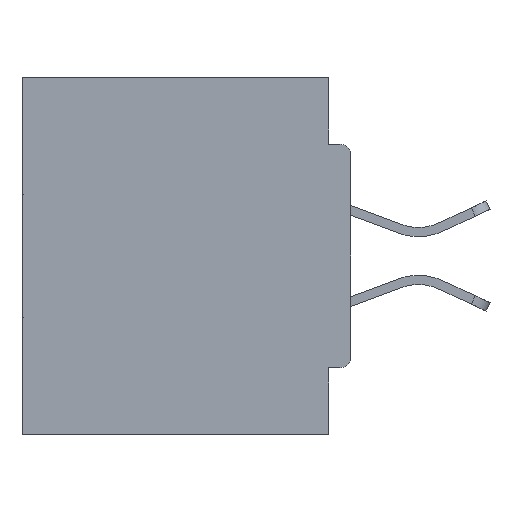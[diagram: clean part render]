
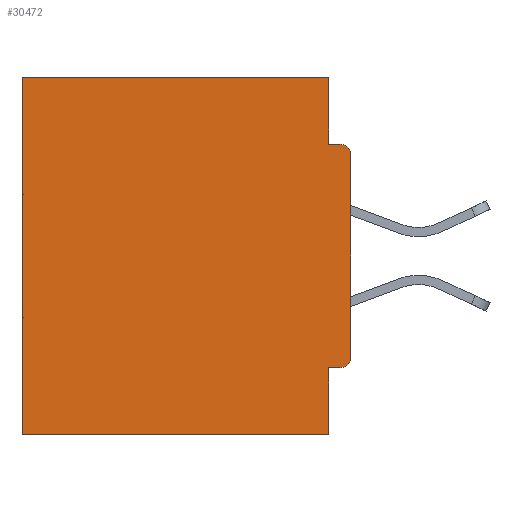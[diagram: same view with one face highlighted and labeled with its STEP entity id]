
A CAD part, left-side view. The second image highlights one B-rep face of the part: STEP entity #30472.
In plain terms, the highlighted planar face has unit normal (-1, 0, 0).
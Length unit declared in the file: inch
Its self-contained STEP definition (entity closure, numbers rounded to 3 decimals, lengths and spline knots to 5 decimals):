
#907 = CARTESIAN_POINT ( 'NONE',  ( 0.298, 0., -0.3915 ) ) ;
#1458 = DIRECTION ( 'NONE',  ( 0., 1., 0. ) ) ;
#2212 = CARTESIAN_POINT ( 'NONE',  ( 0.298, 0.46, 0. ) ) ;
#2393 = CARTESIAN_POINT ( 'NONE',  ( 0.298, 0., -0.1085 ) ) ;
#3038 = CARTESIAN_POINT ( 'NONE',  ( 0.298, 0.015, -0.3915 ) ) ;
#3101 = EDGE_CURVE ( 'NONE', #22892, #24254, #41037, .T. ) ;
#3118 = LINE ( 'NONE', #23529, #28867 ) ;
#4680 = DIRECTION ( 'NONE',  ( 0., 1., 0. ) ) ;
#4734 = EDGE_CURVE ( 'NONE', #29090, #37944, #10026, .T. ) ;
#5075 = DIRECTION ( 'NONE',  ( 0., 0., -1. ) ) ;
#5515 = CIRCLE ( 'NONE', #8658, 0.015 ) ;
#5885 = ORIENTED_EDGE ( 'NONE', *, *, #31345, .F. ) ;
#6039 = CIRCLE ( 'NONE', #16067, 0.015 ) ;
#6059 = CARTESIAN_POINT ( 'NONE',  ( 0.298, 0., 0. ) ) ;
#6969 = CARTESIAN_POINT ( 'NONE',  ( 0.298, 0., 0. ) ) ;
#8136 = CARTESIAN_POINT ( 'NONE',  ( 0.298, 0.015, -0.4065 ) ) ;
#8409 = CARTESIAN_POINT ( 'NONE',  ( 0.298, 0.031, -0.5 ) ) ;
#8658 = AXIS2_PLACEMENT_3D ( 'NONE', #3038, #28784, #19251 ) ;
#8684 = CARTESIAN_POINT ( 'NONE',  ( 0.298, 0.031, -0.4065 ) ) ;
#9141 = VECTOR ( 'NONE', #19854, 39.37008 ) ;
#9294 = CARTESIAN_POINT ( 'NONE',  ( 0.298, 0.015, -0.1085 ) ) ;
#9324 = DIRECTION ( 'NONE',  ( 0., 0., -1. ) ) ;
#9918 = CARTESIAN_POINT ( 'NONE',  ( 0.298, 0.031, -0.5 ) ) ;
#10026 = LINE ( 'NONE', #22534, #19317 ) ;
#10272 = ORIENTED_EDGE ( 'NONE', *, *, #3101, .F. ) ;
#10493 = VERTEX_POINT ( 'NONE', #907 ) ;
#12898 = CARTESIAN_POINT ( 'NONE',  ( 0.298, 0., 0. ) ) ;
#12984 = EDGE_CURVE ( 'NONE', #40757, #29732, #6039, .T. ) ;
#13037 = DIRECTION ( 'NONE',  ( 0., 1., 0. ) ) ;
#13090 = ORIENTED_EDGE ( 'NONE', *, *, #30831, .F. ) ;
#13136 = EDGE_CURVE ( 'NONE', #22892, #10493, #5515, .T. ) ;
#13791 = VECTOR ( 'NONE', #9324, 39.37008 ) ;
#14274 = CARTESIAN_POINT ( 'NONE',  ( 0.298, 0., -0.4065 ) ) ;
#15206 = DIRECTION ( 'NONE',  ( -1., 0., 0. ) ) ;
#15630 = CARTESIAN_POINT ( 'NONE',  ( 0.298, 0.015, -0.0935 ) ) ;
#16067 = AXIS2_PLACEMENT_3D ( 'NONE', #9294, #15206, #41943 ) ;
#16586 = DIRECTION ( 'NONE',  ( 0., 0., -1. ) ) ;
#17011 = PLANE ( 'NONE',  #21272 ) ;
#17064 = ORIENTED_EDGE ( 'NONE', *, *, #37421, .T. ) ;
#17360 = LINE ( 'NONE', #9918, #9141 ) ;
#17787 = ORIENTED_EDGE ( 'NONE', *, *, #29115, .F. ) ;
#17821 = ORIENTED_EDGE ( 'NONE', *, *, #20312, .F. ) ;
#19251 = DIRECTION ( 'NONE',  ( 0., 0., -1. ) ) ;
#19317 = VECTOR ( 'NONE', #31996, 39.37008 ) ;
#19500 = CARTESIAN_POINT ( 'NONE',  ( 0.298, 0.46, -0.5 ) ) ;
#19854 = DIRECTION ( 'NONE',  ( 0., 0., -1. ) ) ;
#20312 = EDGE_CURVE ( 'NONE', #24254, #35761, #17360, .T. ) ;
#21272 = AXIS2_PLACEMENT_3D ( 'NONE', #6969, #29721, #16586 ) ;
#22534 = CARTESIAN_POINT ( 'NONE',  ( 0.298, 0.46, 0. ) ) ;
#22892 = VERTEX_POINT ( 'NONE', #8136 ) ;
#22915 = VERTEX_POINT ( 'NONE', #27572 ) ;
#23529 = CARTESIAN_POINT ( 'NONE',  ( 0.298, 0., -0.0935 ) ) ;
#24254 = VERTEX_POINT ( 'NONE', #8684 ) ;
#24316 = CARTESIAN_POINT ( 'NONE',  ( 0.298, 0., -0.5 ) ) ;
#24353 = ORIENTED_EDGE ( 'NONE', *, *, #36372, .F. ) ;
#24803 = CARTESIAN_POINT ( 'NONE',  ( 0.298, 0.031, -0.5 ) ) ;
#26842 = DIRECTION ( 'NONE',  ( 0., -1., 0. ) ) ;
#27101 = ORIENTED_EDGE ( 'NONE', *, *, #4734, .T. ) ;
#27228 = LINE ( 'NONE', #12898, #32347 ) ;
#27572 = CARTESIAN_POINT ( 'NONE',  ( 0.298, 0.031, -0.0935 ) ) ;
#28109 = FACE_OUTER_BOUND ( 'NONE', #30601, .T. ) ;
#28784 = DIRECTION ( 'NONE',  ( -1., 0., 0. ) ) ;
#28867 = VECTOR ( 'NONE', #26842, 39.37008 ) ;
#29090 = VERTEX_POINT ( 'NONE', #2212 ) ;
#29115 = EDGE_CURVE ( 'NONE', #40757, #10493, #29824, .T. ) ;
#29721 = DIRECTION ( 'NONE',  ( 1., 0., 0. ) ) ;
#29732 = VERTEX_POINT ( 'NONE', #15630 ) ;
#29824 = LINE ( 'NONE', #6059, #13791 ) ;
#30472 = ADVANCED_FACE ( 'NONE', ( #28109 ), #17011, .F. ) ;
#30561 = LINE ( 'NONE', #24316, #39222 ) ;
#30601 = EDGE_LOOP ( 'NONE', ( #40953, #24353, #13090, #17064, #27101, #5885, #17821, #10272, #41126, #17787 ) ) ;
#30831 = EDGE_CURVE ( 'NONE', #33313, #22915, #34707, .T. ) ;
#31345 = EDGE_CURVE ( 'NONE', #35761, #37944, #30561, .T. ) ;
#31996 = DIRECTION ( 'NONE',  ( 0., 0., -1. ) ) ;
#32271 = CARTESIAN_POINT ( 'NONE',  ( 0.298, 0.031, 0. ) ) ;
#32347 = VECTOR ( 'NONE', #13037, 39.37008 ) ;
#33313 = VERTEX_POINT ( 'NONE', #32271 ) ;
#34707 = LINE ( 'NONE', #24803, #42359 ) ;
#35761 = VERTEX_POINT ( 'NONE', #8409 ) ;
#36372 = EDGE_CURVE ( 'NONE', #22915, #29732, #3118, .T. ) ;
#37421 = EDGE_CURVE ( 'NONE', #33313, #29090, #27228, .T. ) ;
#37944 = VERTEX_POINT ( 'NONE', #19500 ) ;
#39222 = VECTOR ( 'NONE', #1458, 39.37008 ) ;
#40524 = VECTOR ( 'NONE', #4680, 39.37008 ) ;
#40757 = VERTEX_POINT ( 'NONE', #2393 ) ;
#40953 = ORIENTED_EDGE ( 'NONE', *, *, #12984, .T. ) ;
#41037 = LINE ( 'NONE', #14274, #40524 ) ;
#41126 = ORIENTED_EDGE ( 'NONE', *, *, #13136, .T. ) ;
#41943 = DIRECTION ( 'NONE',  ( 0., 0., -1. ) ) ;
#42359 = VECTOR ( 'NONE', #5075, 39.37008 ) ;
